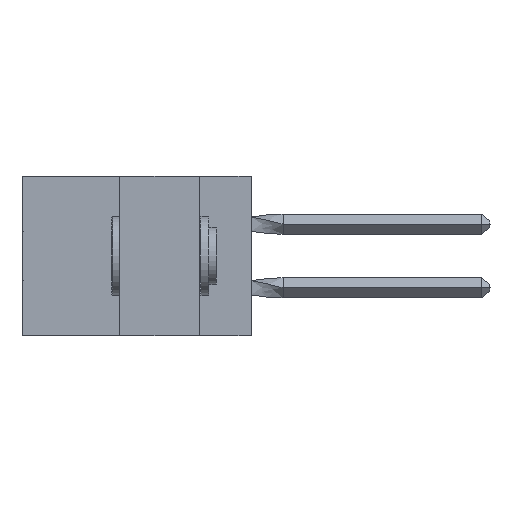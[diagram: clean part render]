
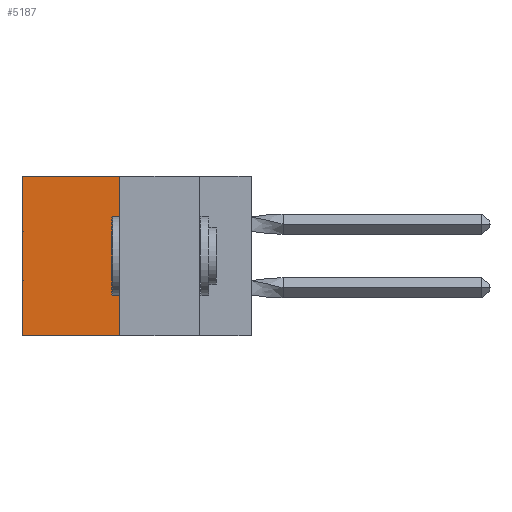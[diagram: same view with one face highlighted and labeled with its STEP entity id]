
A CAD part, left-side view. The second image highlights one B-rep face of the part: STEP entity #5187.
In plain terms, the highlighted planar face has unit normal (-1, 0, 0).
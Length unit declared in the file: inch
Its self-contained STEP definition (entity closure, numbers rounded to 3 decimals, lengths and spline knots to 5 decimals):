
#243 = ORIENTED_EDGE ( 'NONE', *, *, #4136, .F. ) ;
#3759 = CARTESIAN_POINT ( 'NONE',  ( 0.305, 0.413, 0. ) ) ;
#3917 = CARTESIAN_POINT ( 'NONE',  ( 0.305, 0.413, -0.5 ) ) ;
#4136 = EDGE_CURVE ( 'NONE', #41098, #25573, #8540, .T. ) ;
#4839 = LINE ( 'NONE', #3759, #21358 ) ;
#5187 = ADVANCED_FACE ( 'NONE', ( #9064 ), #21078, .F. ) ;
#6470 = ORIENTED_EDGE ( 'NONE', *, *, #15018, .T. ) ;
#6734 = DIRECTION ( 'NONE',  ( 0., 0., -1. ) ) ;
#8113 = ORIENTED_EDGE ( 'NONE', *, *, #30225, .F. ) ;
#8210 = DIRECTION ( 'NONE',  ( 0., 0., -1. ) ) ;
#8540 = LINE ( 'NONE', #34490, #10737 ) ;
#9064 = FACE_OUTER_BOUND ( 'NONE', #36111, .T. ) ;
#10737 = VECTOR ( 'NONE', #6734, 39.37008 ) ;
#14956 = VECTOR ( 'NONE', #44444, 39.37008 ) ;
#15018 = EDGE_CURVE ( 'NONE', #39517, #18620, #25714, .T. ) ;
#15238 = VECTOR ( 'NONE', #8210, 39.37008 ) ;
#15738 = CARTESIAN_POINT ( 'NONE',  ( 0.305, 0.413, 0. ) ) ;
#18349 = CARTESIAN_POINT ( 'NONE',  ( 0.305, 0.72, -0.5 ) ) ;
#18620 = VERTEX_POINT ( 'NONE', #28079 ) ;
#19212 = EDGE_CURVE ( 'NONE', #41098, #39517, #4839, .T. ) ;
#21078 = PLANE ( 'NONE',  #34214 ) ;
#21358 = VECTOR ( 'NONE', #32049, 39.37008 ) ;
#22168 = LINE ( 'NONE', #27080, #14956 ) ;
#25573 = VERTEX_POINT ( 'NONE', #3917 ) ;
#25714 = LINE ( 'NONE', #18349, #15238 ) ;
#27080 = CARTESIAN_POINT ( 'NONE',  ( 0.305, 0.413, -0.5 ) ) ;
#28079 = CARTESIAN_POINT ( 'NONE',  ( 0.305, 0.72, -0.5 ) ) ;
#28904 = DIRECTION ( 'NONE',  ( 1., 0., 0. ) ) ;
#29508 = CARTESIAN_POINT ( 'NONE',  ( 0.305, 0.413, -0.5 ) ) ;
#30225 = EDGE_CURVE ( 'NONE', #25573, #18620, #22168, .T. ) ;
#31784 = CARTESIAN_POINT ( 'NONE',  ( 0.305, 0.72, 0. ) ) ;
#32049 = DIRECTION ( 'NONE',  ( 0., 1., 0. ) ) ;
#32596 = DIRECTION ( 'NONE',  ( 0., 0., -1. ) ) ;
#34214 = AXIS2_PLACEMENT_3D ( 'NONE', #29508, #28904, #32596 ) ;
#34490 = CARTESIAN_POINT ( 'NONE',  ( 0.305, 0.413, -0.5 ) ) ;
#36111 = EDGE_LOOP ( 'NONE', ( #6470, #8113, #243, #41207 ) ) ;
#39517 = VERTEX_POINT ( 'NONE', #31784 ) ;
#41098 = VERTEX_POINT ( 'NONE', #15738 ) ;
#41207 = ORIENTED_EDGE ( 'NONE', *, *, #19212, .T. ) ;
#44444 = DIRECTION ( 'NONE',  ( 0., 1., 0. ) ) ;
